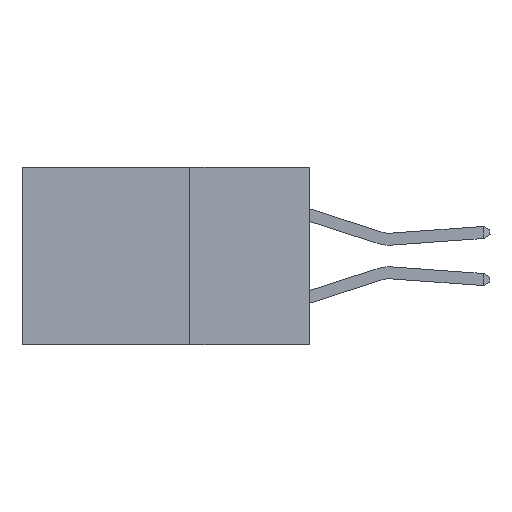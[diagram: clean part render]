
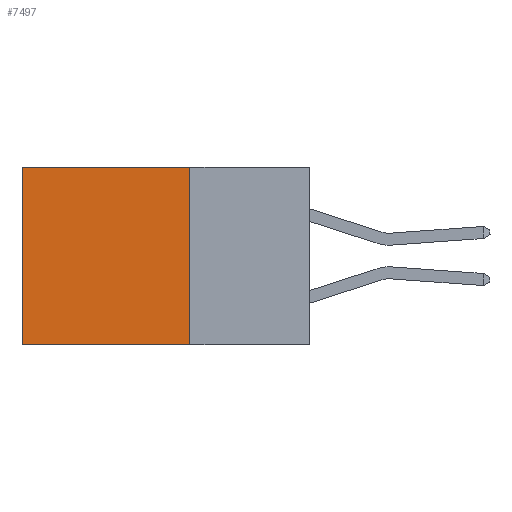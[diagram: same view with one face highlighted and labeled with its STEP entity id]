
A CAD part, left-side view. The second image highlights one B-rep face of the part: STEP entity #7497.
In plain terms, the highlighted planar face has unit normal (-1, 0, 0).
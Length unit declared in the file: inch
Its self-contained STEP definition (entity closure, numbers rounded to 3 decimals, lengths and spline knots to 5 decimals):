
#130 = VERTEX_POINT ( 'NONE', #2939 ) ;
#203 = EDGE_CURVE ( 'NONE', #8638, #130, #4043, .T. ) ;
#629 = PLANE ( 'NONE',  #10384 ) ;
#1366 = CARTESIAN_POINT ( 'NONE',  ( 0.298, 0.25, 0. ) ) ;
#1498 = DIRECTION ( 'NONE',  ( 1., 0., 0. ) ) ;
#1775 = LINE ( 'NONE', #3933, #10599 ) ;
#2939 = CARTESIAN_POINT ( 'NONE',  ( 0.298, 0.25, -0.37 ) ) ;
#3033 = EDGE_CURVE ( 'NONE', #9575, #9243, #9951, .T. ) ;
#3331 = DIRECTION ( 'NONE',  ( 0., 1., 0. ) ) ;
#3933 = CARTESIAN_POINT ( 'NONE',  ( 0.298, 0.25, 0. ) ) ;
#4017 = LINE ( 'NONE', #8631, #5117 ) ;
#4043 = LINE ( 'NONE', #9689, #6349 ) ;
#4881 = CARTESIAN_POINT ( 'NONE',  ( 0.298, 0.25, 0. ) ) ;
#5029 = EDGE_LOOP ( 'NONE', ( #7105, #7397, #7157, #10054 ) ) ;
#5117 = VECTOR ( 'NONE', #3331, 39.37008 ) ;
#5765 = DIRECTION ( 'NONE',  ( 0., 1., 0. ) ) ;
#6349 = VECTOR ( 'NONE', #7201, 39.37008 ) ;
#6458 = EDGE_CURVE ( 'NONE', #130, #9243, #4017, .T. ) ;
#7088 = CARTESIAN_POINT ( 'NONE',  ( 0.298, 0.6, 0. ) ) ;
#7105 = ORIENTED_EDGE ( 'NONE', *, *, #3033, .T. ) ;
#7157 = ORIENTED_EDGE ( 'NONE', *, *, #203, .F. ) ;
#7201 = DIRECTION ( 'NONE',  ( 0., 0., -1. ) ) ;
#7397 = ORIENTED_EDGE ( 'NONE', *, *, #6458, .F. ) ;
#7490 = DIRECTION ( 'NONE',  ( 0., 0., -1. ) ) ;
#7497 = ADVANCED_FACE ( 'NONE', ( #9294 ), #629, .F. ) ;
#8328 = VECTOR ( 'NONE', #10374, 39.37008 ) ;
#8597 = CARTESIAN_POINT ( 'NONE',  ( 0.298, 0.6, 0. ) ) ;
#8631 = CARTESIAN_POINT ( 'NONE',  ( 0.298, 0.25, -0.37 ) ) ;
#8638 = VERTEX_POINT ( 'NONE', #1366 ) ;
#9102 = CARTESIAN_POINT ( 'NONE',  ( 0.298, 0.6, -0.37 ) ) ;
#9243 = VERTEX_POINT ( 'NONE', #9102 ) ;
#9294 = FACE_OUTER_BOUND ( 'NONE', #5029, .T. ) ;
#9575 = VERTEX_POINT ( 'NONE', #7088 ) ;
#9689 = CARTESIAN_POINT ( 'NONE',  ( 0.298, 0.25, 0. ) ) ;
#9951 = LINE ( 'NONE', #8597, #8328 ) ;
#10054 = ORIENTED_EDGE ( 'NONE', *, *, #10304, .T. ) ;
#10304 = EDGE_CURVE ( 'NONE', #8638, #9575, #1775, .T. ) ;
#10374 = DIRECTION ( 'NONE',  ( 0., 0., -1. ) ) ;
#10384 = AXIS2_PLACEMENT_3D ( 'NONE', #4881, #1498, #7490 ) ;
#10599 = VECTOR ( 'NONE', #5765, 39.37008 ) ;
